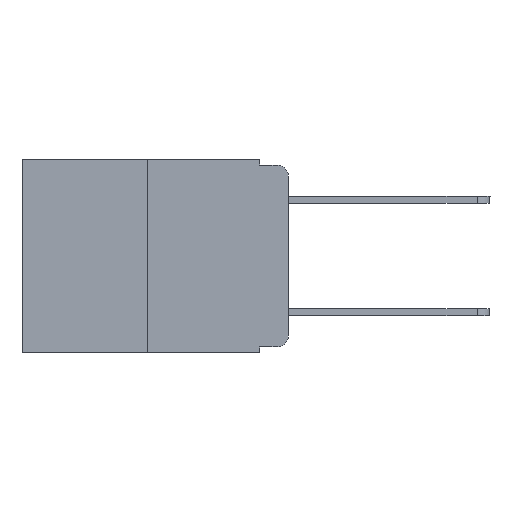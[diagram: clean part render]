
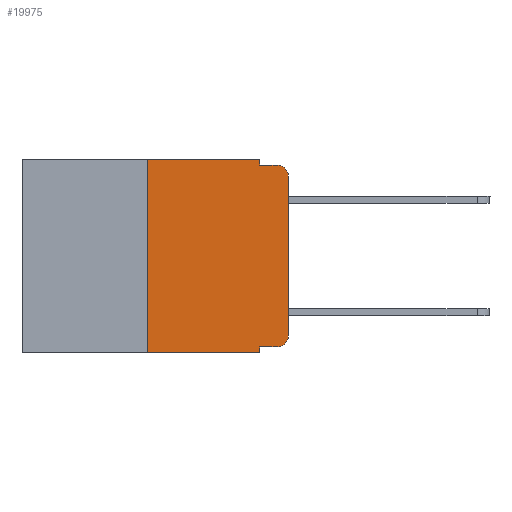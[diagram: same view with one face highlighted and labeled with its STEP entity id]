
A CAD part, left-side view. The second image highlights one B-rep face of the part: STEP entity #19975.
In plain terms, the highlighted planar face has unit normal (-1, 0, 0).
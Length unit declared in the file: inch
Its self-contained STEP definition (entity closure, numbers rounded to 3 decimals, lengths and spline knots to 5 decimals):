
#17 = DIRECTION ( 'NONE',  ( 0., -1., 0. ) ) ;
#522 = EDGE_CURVE ( 'NONE', #3059, #4557, #18921, .T. ) ;
#557 = DIRECTION ( 'NONE',  ( 1., 0., 0. ) ) ;
#614 = VECTOR ( 'NONE', #14470, 39.37008 ) ;
#879 = DIRECTION ( 'NONE',  ( 0., -1., 0. ) ) ;
#1164 = ORIENTED_EDGE ( 'NONE', *, *, #10695, .T. ) ;
#1205 = CARTESIAN_POINT ( 'NONE',  ( 0., 0.02, -0.333 ) ) ;
#1799 = VECTOR ( 'NONE', #20446, 39.37008 ) ;
#1931 = EDGE_CURVE ( 'NONE', #16536, #18602, #5567, .T. ) ;
#2379 = CARTESIAN_POINT ( 'NONE',  ( 0., 0.473, 0. ) ) ;
#3059 = VERTEX_POINT ( 'NONE', #1205 ) ;
#3224 = EDGE_CURVE ( 'NONE', #16437, #18602, #5913, .T. ) ;
#3228 = EDGE_CURVE ( 'NONE', #8691, #16536, #13686, .T. ) ;
#3292 = CARTESIAN_POINT ( 'NONE',  ( 0., 0., -0.313 ) ) ;
#3522 = DIRECTION ( 'NONE',  ( 0., 0., -1. ) ) ;
#4191 = DIRECTION ( 'NONE',  ( 0., 0., -1. ) ) ;
#4292 = ORIENTED_EDGE ( 'NONE', *, *, #21021, .F. ) ;
#4420 = CARTESIAN_POINT ( 'NONE',  ( 0., 0.051, -0.343 ) ) ;
#4557 = VERTEX_POINT ( 'NONE', #3292 ) ;
#5567 = LINE ( 'NONE', #15501, #21627 ) ;
#5670 = ORIENTED_EDGE ( 'NONE', *, *, #18056, .F. ) ;
#5913 = CIRCLE ( 'NONE', #20343, 0.02 ) ;
#6136 = EDGE_CURVE ( 'NONE', #4557, #16437, #24565, .T. ) ;
#6749 = CARTESIAN_POINT ( 'NONE',  ( 0., 0.051, -0.333 ) ) ;
#6930 = CARTESIAN_POINT ( 'NONE',  ( 0., 0.473, -0.343 ) ) ;
#7939 = VERTEX_POINT ( 'NONE', #4420 ) ;
#8416 = EDGE_LOOP ( 'NONE', ( #17177, #21604, #12184, #23189, #4292, #5670, #1164, #17769, #22273, #21103 ) ) ;
#8603 = LINE ( 'NONE', #24355, #14681 ) ;
#8691 = VERTEX_POINT ( 'NONE', #15703 ) ;
#8847 = AXIS2_PLACEMENT_3D ( 'NONE', #2379, #557, #10217 ) ;
#9002 = AXIS2_PLACEMENT_3D ( 'NONE', #13972, #24022, #20164 ) ;
#9676 = DIRECTION ( 'NONE',  ( 0., 0., -1. ) ) ;
#10217 = DIRECTION ( 'NONE',  ( 0., 0., -1. ) ) ;
#10695 = EDGE_CURVE ( 'NONE', #23077, #7939, #24614, .T. ) ;
#12184 = ORIENTED_EDGE ( 'NONE', *, *, #1931, .F. ) ;
#12281 = FACE_OUTER_BOUND ( 'NONE', #8416, .T. ) ;
#12484 = VECTOR ( 'NONE', #9676, 39.37008 ) ;
#12606 = CARTESIAN_POINT ( 'NONE',  ( 0., 0.051, -0.333 ) ) ;
#12688 = CARTESIAN_POINT ( 'NONE',  ( 0., 0., -0.03 ) ) ;
#13229 = VECTOR ( 'NONE', #14803, 39.37008 ) ;
#13686 = LINE ( 'NONE', #15243, #12484 ) ;
#13826 = CARTESIAN_POINT ( 'NONE',  ( 0., 0.02, -0.03 ) ) ;
#13838 = VERTEX_POINT ( 'NONE', #12606 ) ;
#13972 = CARTESIAN_POINT ( 'NONE',  ( 0., 0.02, -0.313 ) ) ;
#14470 = DIRECTION ( 'NONE',  ( 0., 0., 1. ) ) ;
#14621 = PLANE ( 'NONE',  #8847 ) ;
#14634 = DIRECTION ( 'NONE',  ( 0., -1., 0. ) ) ;
#14681 = VECTOR ( 'NONE', #879, 39.37008 ) ;
#14803 = DIRECTION ( 'NONE',  ( 0., -1., 0. ) ) ;
#15104 = EDGE_CURVE ( 'NONE', #13838, #3059, #24430, .T. ) ;
#15243 = CARTESIAN_POINT ( 'NONE',  ( 0., 0.051, 0. ) ) ;
#15501 = CARTESIAN_POINT ( 'NONE',  ( 0., 0.051, -0.01 ) ) ;
#15703 = CARTESIAN_POINT ( 'NONE',  ( 0., 0.051, 0. ) ) ;
#16176 = EDGE_CURVE ( 'NONE', #13838, #7939, #19804, .T. ) ;
#16437 = VERTEX_POINT ( 'NONE', #12688 ) ;
#16536 = VERTEX_POINT ( 'NONE', #19399 ) ;
#16800 = CARTESIAN_POINT ( 'NONE',  ( 0., 0.25, -0.343 ) ) ;
#17177 = ORIENTED_EDGE ( 'NONE', *, *, #6136, .T. ) ;
#17326 = DIRECTION ( 'NONE',  ( -1., 0., 0. ) ) ;
#17769 = ORIENTED_EDGE ( 'NONE', *, *, #16176, .F. ) ;
#17991 = LINE ( 'NONE', #24412, #614 ) ;
#18056 = EDGE_CURVE ( 'NONE', #23077, #23915, #17991, .T. ) ;
#18134 = CARTESIAN_POINT ( 'NONE',  ( 0., 0.051, 0. ) ) ;
#18231 = CARTESIAN_POINT ( 'NONE',  ( 0., 0., 0. ) ) ;
#18602 = VERTEX_POINT ( 'NONE', #23418 ) ;
#18921 = CIRCLE ( 'NONE', #9002, 0.02 ) ;
#19399 = CARTESIAN_POINT ( 'NONE',  ( 0., 0.051, -0.01 ) ) ;
#19804 = LINE ( 'NONE', #18134, #19886 ) ;
#19886 = VECTOR ( 'NONE', #4191, 39.37008 ) ;
#19975 = ADVANCED_FACE ( 'NONE', ( #12281 ), #14621, .F. ) ;
#20164 = DIRECTION ( 'NONE',  ( 0., 0., -1. ) ) ;
#20343 = AXIS2_PLACEMENT_3D ( 'NONE', #13826, #17326, #3522 ) ;
#20446 = DIRECTION ( 'NONE',  ( 0., 0., 1. ) ) ;
#21021 = EDGE_CURVE ( 'NONE', #23915, #8691, #8603, .T. ) ;
#21103 = ORIENTED_EDGE ( 'NONE', *, *, #522, .T. ) ;
#21604 = ORIENTED_EDGE ( 'NONE', *, *, #3224, .T. ) ;
#21627 = VECTOR ( 'NONE', #17, 39.37008 ) ;
#22273 = ORIENTED_EDGE ( 'NONE', *, *, #15104, .T. ) ;
#23077 = VERTEX_POINT ( 'NONE', #16800 ) ;
#23189 = ORIENTED_EDGE ( 'NONE', *, *, #3228, .F. ) ;
#23418 = CARTESIAN_POINT ( 'NONE',  ( 0., 0.02, -0.01 ) ) ;
#23915 = VERTEX_POINT ( 'NONE', #24965 ) ;
#24022 = DIRECTION ( 'NONE',  ( -1., 0., 0. ) ) ;
#24355 = CARTESIAN_POINT ( 'NONE',  ( 0., 0.473, 0. ) ) ;
#24412 = CARTESIAN_POINT ( 'NONE',  ( 0., 0.25, 0. ) ) ;
#24430 = LINE ( 'NONE', #6749, #24499 ) ;
#24499 = VECTOR ( 'NONE', #14634, 39.37008 ) ;
#24565 = LINE ( 'NONE', #18231, #1799 ) ;
#24614 = LINE ( 'NONE', #6930, #13229 ) ;
#24965 = CARTESIAN_POINT ( 'NONE',  ( 0., 0.25, 0. ) ) ;
